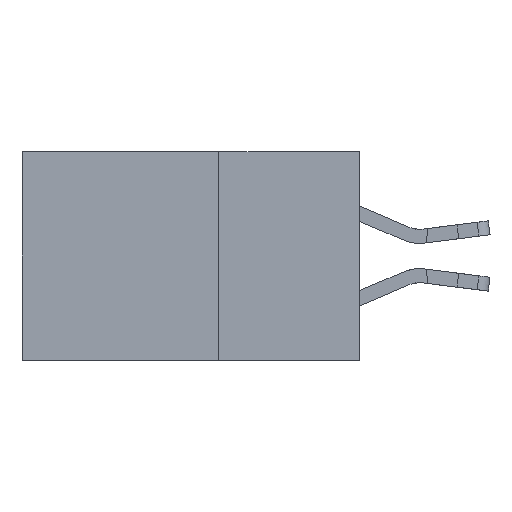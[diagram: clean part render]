
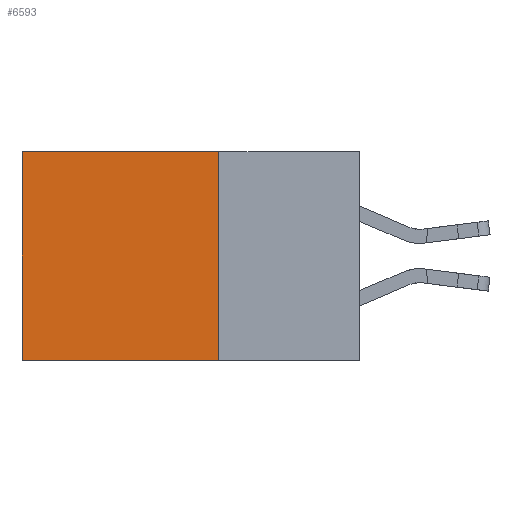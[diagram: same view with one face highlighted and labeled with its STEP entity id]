
A CAD part, left-side view. The second image highlights one B-rep face of the part: STEP entity #6593.
In plain terms, the highlighted planar face has unit normal (-1, 0, 0).
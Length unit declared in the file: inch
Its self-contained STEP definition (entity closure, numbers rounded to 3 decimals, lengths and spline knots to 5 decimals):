
#678 = VECTOR ( 'NONE', #22187, 39.37008 ) ;
#1415 = LINE ( 'NONE', #22352, #14738 ) ;
#1891 = VERTEX_POINT ( 'NONE', #19452 ) ;
#2046 = ORIENTED_EDGE ( 'NONE', *, *, #20270, .F. ) ;
#3329 = VERTEX_POINT ( 'NONE', #8033 ) ;
#3869 = CARTESIAN_POINT ( 'NONE',  ( 0.2875, 0.25, 0. ) ) ;
#4273 = AXIS2_PLACEMENT_3D ( 'NONE', #3869, #11513, #9739 ) ;
#5297 = DIRECTION ( 'NONE',  ( 0., 1., 0. ) ) ;
#6593 = ADVANCED_FACE ( 'NONE', ( #16982 ), #13617, .F. ) ;
#6862 = DIRECTION ( 'NONE',  ( 0., 1., 0. ) ) ;
#7113 = LINE ( 'NONE', #23932, #678 ) ;
#7405 = ORIENTED_EDGE ( 'NONE', *, *, #14008, .F. ) ;
#7962 = EDGE_CURVE ( 'NONE', #24155, #7998, #1415, .T. ) ;
#7998 = VERTEX_POINT ( 'NONE', #23334 ) ;
#8033 = CARTESIAN_POINT ( 'NONE',  ( 0.2875, 0.6, -0.37 ) ) ;
#8505 = CARTESIAN_POINT ( 'NONE',  ( 0.2875, 0.25, -0.37 ) ) ;
#8611 = VECTOR ( 'NONE', #8742, 39.37008 ) ;
#8742 = DIRECTION ( 'NONE',  ( 0., 0., -1. ) ) ;
#9739 = DIRECTION ( 'NONE',  ( 0., 0., -1. ) ) ;
#11237 = VECTOR ( 'NONE', #6862, 39.37008 ) ;
#11513 = DIRECTION ( 'NONE',  ( 1., 0., 0. ) ) ;
#12561 = EDGE_CURVE ( 'NONE', #7998, #3329, #24047, .T. ) ;
#12618 = CARTESIAN_POINT ( 'NONE',  ( 0.2875, 0.6, 0. ) ) ;
#12624 = LINE ( 'NONE', #8505, #11237 ) ;
#13617 = PLANE ( 'NONE',  #4273 ) ;
#14008 = EDGE_CURVE ( 'NONE', #24155, #1891, #7113, .T. ) ;
#14738 = VECTOR ( 'NONE', #5297, 39.37008 ) ;
#16982 = FACE_OUTER_BOUND ( 'NONE', #24013, .T. ) ;
#17126 = ORIENTED_EDGE ( 'NONE', *, *, #12561, .T. ) ;
#19452 = CARTESIAN_POINT ( 'NONE',  ( 0.2875, 0.25, -0.37 ) ) ;
#20270 = EDGE_CURVE ( 'NONE', #1891, #3329, #12624, .T. ) ;
#20909 = ORIENTED_EDGE ( 'NONE', *, *, #7962, .T. ) ;
#22187 = DIRECTION ( 'NONE',  ( 0., 0., -1. ) ) ;
#22352 = CARTESIAN_POINT ( 'NONE',  ( 0.2875, 0.25, 0. ) ) ;
#23302 = CARTESIAN_POINT ( 'NONE',  ( 0.2875, 0.25, 0. ) ) ;
#23334 = CARTESIAN_POINT ( 'NONE',  ( 0.2875, 0.6, 0. ) ) ;
#23932 = CARTESIAN_POINT ( 'NONE',  ( 0.2875, 0.25, 0. ) ) ;
#24013 = EDGE_LOOP ( 'NONE', ( #17126, #2046, #7405, #20909 ) ) ;
#24047 = LINE ( 'NONE', #12618, #8611 ) ;
#24155 = VERTEX_POINT ( 'NONE', #23302 ) ;
